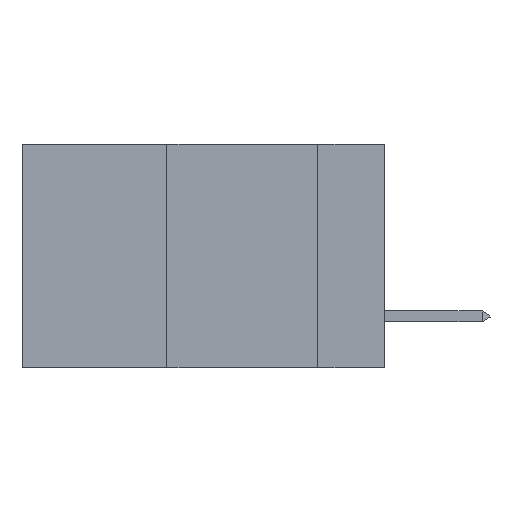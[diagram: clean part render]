
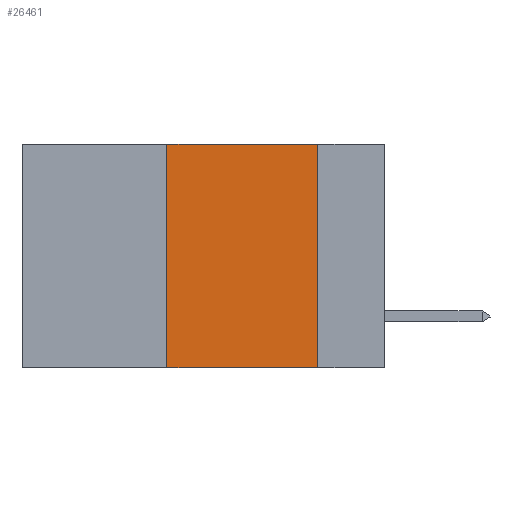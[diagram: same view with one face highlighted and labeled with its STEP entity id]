
A CAD part, left-side view. The second image highlights one B-rep face of the part: STEP entity #26461.
In plain terms, the highlighted planar face has unit normal (-1, 0, 0).
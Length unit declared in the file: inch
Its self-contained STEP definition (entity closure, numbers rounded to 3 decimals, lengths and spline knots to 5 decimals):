
#1220 = ORIENTED_EDGE ( 'NONE', *, *, #15983, .F. ) ;
#1393 = VECTOR ( 'NONE', #16752, 39.37008 ) ;
#2577 = CARTESIAN_POINT ( 'NONE',  ( 0., 0.6, -0.37 ) ) ;
#2856 = DIRECTION ( 'NONE',  ( 0., -1., 0. ) ) ;
#2943 = AXIS2_PLACEMENT_3D ( 'NONE', #8250, #5817, #23076 ) ;
#3333 = CARTESIAN_POINT ( 'NONE',  ( 0., 0.36, -0.37 ) ) ;
#3563 = FACE_OUTER_BOUND ( 'NONE', #5470, .T. ) ;
#3577 = PLANE ( 'NONE',  #2943 ) ;
#3615 = LINE ( 'NONE', #11959, #20227 ) ;
#3704 = VERTEX_POINT ( 'NONE', #9727 ) ;
#4041 = CARTESIAN_POINT ( 'NONE',  ( 0., 0.11, -0.37 ) ) ;
#5470 = EDGE_LOOP ( 'NONE', ( #1220, #15183, #15739, #18318 ) ) ;
#5817 = DIRECTION ( 'NONE',  ( 1., 0., 0. ) ) ;
#6842 = DIRECTION ( 'NONE',  ( 0., -1., 0. ) ) ;
#6981 = CARTESIAN_POINT ( 'NONE',  ( 0., 0.36, 0. ) ) ;
#7038 = LINE ( 'NONE', #9703, #1393 ) ;
#8250 = CARTESIAN_POINT ( 'NONE',  ( 0., 0.6, 0. ) ) ;
#8921 = LINE ( 'NONE', #6981, #9234 ) ;
#9234 = VECTOR ( 'NONE', #26106, 39.37008 ) ;
#9703 = CARTESIAN_POINT ( 'NONE',  ( 0., 0.11, 0. ) ) ;
#9727 = CARTESIAN_POINT ( 'NONE',  ( 0., 0.11, 0. ) ) ;
#10282 = EDGE_CURVE ( 'NONE', #24995, #3704, #3615, .T. ) ;
#11959 = CARTESIAN_POINT ( 'NONE',  ( 0., 0.6, 0. ) ) ;
#12845 = EDGE_CURVE ( 'NONE', #25670, #26597, #24764, .T. ) ;
#15183 = ORIENTED_EDGE ( 'NONE', *, *, #10282, .F. ) ;
#15739 = ORIENTED_EDGE ( 'NONE', *, *, #19000, .F. ) ;
#15983 = EDGE_CURVE ( 'NONE', #3704, #26597, #7038, .T. ) ;
#16752 = DIRECTION ( 'NONE',  ( 0., 0., -1. ) ) ;
#18318 = ORIENTED_EDGE ( 'NONE', *, *, #12845, .T. ) ;
#19000 = EDGE_CURVE ( 'NONE', #25670, #24995, #8921, .T. ) ;
#19119 = VECTOR ( 'NONE', #6842, 39.37008 ) ;
#19947 = CARTESIAN_POINT ( 'NONE',  ( 0., 0.36, 0. ) ) ;
#20227 = VECTOR ( 'NONE', #2856, 39.37008 ) ;
#23076 = DIRECTION ( 'NONE',  ( 0., 0., -1. ) ) ;
#24764 = LINE ( 'NONE', #2577, #19119 ) ;
#24995 = VERTEX_POINT ( 'NONE', #19947 ) ;
#25670 = VERTEX_POINT ( 'NONE', #3333 ) ;
#26106 = DIRECTION ( 'NONE',  ( 0., 0., 1. ) ) ;
#26461 = ADVANCED_FACE ( 'NONE', ( #3563 ), #3577, .F. ) ;
#26597 = VERTEX_POINT ( 'NONE', #4041 ) ;
